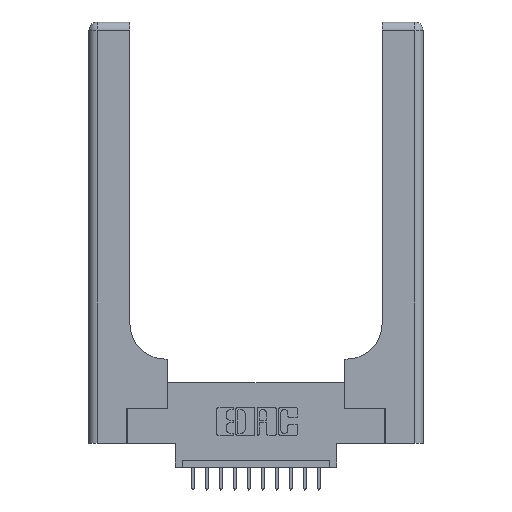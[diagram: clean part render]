
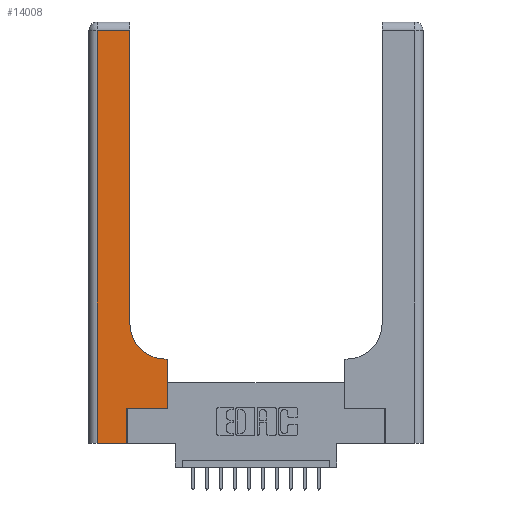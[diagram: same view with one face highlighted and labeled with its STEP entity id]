
A CAD part, top view. The second image highlights one B-rep face of the part: STEP entity #14008.
In plain terms, the highlighted planar face has unit normal (0, 0, 1).
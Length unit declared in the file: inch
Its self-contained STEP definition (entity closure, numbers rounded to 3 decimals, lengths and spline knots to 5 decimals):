
#68 = CARTESIAN_POINT ( 'NONE',  ( 0., 0., 0.37 ) ) ;
#254 = EDGE_CURVE ( 'NONE', #550, #15819, #13075, .T. ) ;
#281 = CARTESIAN_POINT ( 'NONE',  ( 0.5585, 0.25, 0.37 ) ) ;
#341 = VERTEX_POINT ( 'NONE', #14483 ) ;
#394 = CARTESIAN_POINT ( 'NONE',  ( 0.2915, 0.85, 0.37 ) ) ;
#454 = DIRECTION ( 'NONE',  ( 0., 1., 0. ) ) ;
#550 = VERTEX_POINT ( 'NONE', #13280 ) ;
#614 = CARTESIAN_POINT ( 'NONE',  ( 0.269, 0.25, 0.37 ) ) ;
#758 = VERTEX_POINT ( 'NONE', #9192 ) ;
#840 = CARTESIAN_POINT ( 'NONE',  ( 0.06, 3., 0.37 ) ) ;
#1533 = EDGE_CURVE ( 'NONE', #8437, #16231, #4680, .T. ) ;
#2002 = CIRCLE ( 'NONE', #5046, 0.25 ) ;
#2064 = AXIS2_PLACEMENT_3D ( 'NONE', #11415, #4704, #16724 ) ;
#2365 = LINE ( 'NONE', #614, #11298 ) ;
#2386 = ORIENTED_EDGE ( 'NONE', *, *, #16199, .T. ) ;
#2540 = DIRECTION ( 'NONE',  ( -1., 0., 0. ) ) ;
#2705 = EDGE_CURVE ( 'NONE', #16231, #16691, #9404, .T. ) ;
#3150 = DIRECTION ( 'NONE',  ( 1., 0., 0. ) ) ;
#3183 = CARTESIAN_POINT ( 'NONE',  ( 0.06, 0., 0.37 ) ) ;
#3597 = ORIENTED_EDGE ( 'NONE', *, *, #11040, .T. ) ;
#4680 = LINE ( 'NONE', #11966, #14492 ) ;
#4704 = DIRECTION ( 'NONE',  ( 0., 0., -1. ) ) ;
#5046 = AXIS2_PLACEMENT_3D ( 'NONE', #9816, #7017, #16265 ) ;
#5164 = CARTESIAN_POINT ( 'NONE',  ( 0.2915, 0.6, 0.37 ) ) ;
#5245 = ORIENTED_EDGE ( 'NONE', *, *, #254, .T. ) ;
#5682 = CARTESIAN_POINT ( 'NONE',  ( 0.06, 2.94, 0.37 ) ) ;
#5760 = DIRECTION ( 'NONE',  ( 1., 0., 0. ) ) ;
#5787 = ORIENTED_EDGE ( 'NONE', *, *, #11257, .T. ) ;
#5892 = CARTESIAN_POINT ( 'NONE',  ( 0.269, 0.25, 0.37 ) ) ;
#5982 = PLANE ( 'NONE',  #2064 ) ;
#6195 = CARTESIAN_POINT ( 'NONE',  ( 0.269, 0., 0.37 ) ) ;
#6802 = VERTEX_POINT ( 'NONE', #3183 ) ;
#6855 = EDGE_CURVE ( 'NONE', #14884, #758, #13353, .T. ) ;
#7017 = DIRECTION ( 'NONE',  ( 0., 0., -1. ) ) ;
#7560 = VECTOR ( 'NONE', #3150, 39.37008 ) ;
#8419 = VECTOR ( 'NONE', #11592, 39.37008 ) ;
#8437 = VERTEX_POINT ( 'NONE', #394 ) ;
#8656 = CARTESIAN_POINT ( 'NONE',  ( 0.2915, 2.94, 0.37 ) ) ;
#9175 = CARTESIAN_POINT ( 'NONE',  ( 0., 2.94, 0.37 ) ) ;
#9181 = ORIENTED_EDGE ( 'NONE', *, *, #2705, .T. ) ;
#9192 = CARTESIAN_POINT ( 'NONE',  ( 0.5415, 0.6, 0.37 ) ) ;
#9207 = VECTOR ( 'NONE', #10533, 39.37008 ) ;
#9404 = LINE ( 'NONE', #9175, #9207 ) ;
#9450 = CARTESIAN_POINT ( 'NONE',  ( 0.5585, 0.6, 0.37 ) ) ;
#9743 = ORIENTED_EDGE ( 'NONE', *, *, #10357, .T. ) ;
#9816 = CARTESIAN_POINT ( 'NONE',  ( 0.5415, 0.85, 0.37 ) ) ;
#10357 = EDGE_CURVE ( 'NONE', #16691, #6802, #12413, .T. ) ;
#10533 = DIRECTION ( 'NONE',  ( -1., 0., 0. ) ) ;
#10713 = FACE_OUTER_BOUND ( 'NONE', #14296, .T. ) ;
#11040 = EDGE_CURVE ( 'NONE', #6802, #550, #12604, .T. ) ;
#11257 = EDGE_CURVE ( 'NONE', #341, #14884, #16382, .T. ) ;
#11298 = VECTOR ( 'NONE', #5760, 39.37008 ) ;
#11415 = CARTESIAN_POINT ( 'NONE',  ( 0., 3., 0.37 ) ) ;
#11592 = DIRECTION ( 'NONE',  ( 0., -1., 0. ) ) ;
#11966 = CARTESIAN_POINT ( 'NONE',  ( 0.2915, 3., 0.37 ) ) ;
#12177 = VECTOR ( 'NONE', #454, 39.37008 ) ;
#12413 = LINE ( 'NONE', #840, #8419 ) ;
#12604 = LINE ( 'NONE', #68, #7560 ) ;
#13075 = LINE ( 'NONE', #6195, #13287 ) ;
#13280 = CARTESIAN_POINT ( 'NONE',  ( 0.269, 0., 0.37 ) ) ;
#13287 = VECTOR ( 'NONE', #16872, 39.37008 ) ;
#13353 = LINE ( 'NONE', #5164, #13572 ) ;
#13365 = ORIENTED_EDGE ( 'NONE', *, *, #1533, .T. ) ;
#13572 = VECTOR ( 'NONE', #2540, 39.37008 ) ;
#13681 = ORIENTED_EDGE ( 'NONE', *, *, #6855, .T. ) ;
#13815 = EDGE_CURVE ( 'NONE', #758, #8437, #2002, .T. ) ;
#14008 = ADVANCED_FACE ( 'NONE', ( #10713 ), #5982, .F. ) ;
#14296 = EDGE_LOOP ( 'NONE', ( #13365, #9181, #9743, #3597, #5245, #2386, #5787, #13681, #14512 ) ) ;
#14483 = CARTESIAN_POINT ( 'NONE',  ( 0.5585, 0.25, 0.37 ) ) ;
#14492 = VECTOR ( 'NONE', #14652, 39.37008 ) ;
#14512 = ORIENTED_EDGE ( 'NONE', *, *, #13815, .T. ) ;
#14652 = DIRECTION ( 'NONE',  ( 0., 1., 0. ) ) ;
#14884 = VERTEX_POINT ( 'NONE', #9450 ) ;
#15819 = VERTEX_POINT ( 'NONE', #5892 ) ;
#16199 = EDGE_CURVE ( 'NONE', #15819, #341, #2365, .T. ) ;
#16231 = VERTEX_POINT ( 'NONE', #8656 ) ;
#16265 = DIRECTION ( 'NONE',  ( 1., 0., 0. ) ) ;
#16382 = LINE ( 'NONE', #281, #12177 ) ;
#16691 = VERTEX_POINT ( 'NONE', #5682 ) ;
#16724 = DIRECTION ( 'NONE',  ( -1., 0., 0. ) ) ;
#16872 = DIRECTION ( 'NONE',  ( 0., 1., 0. ) ) ;
